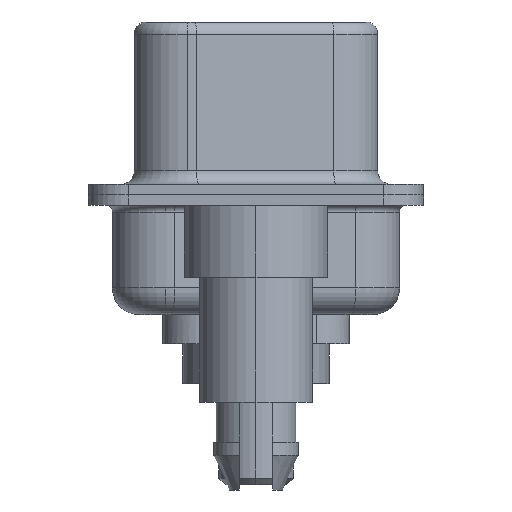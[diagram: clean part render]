
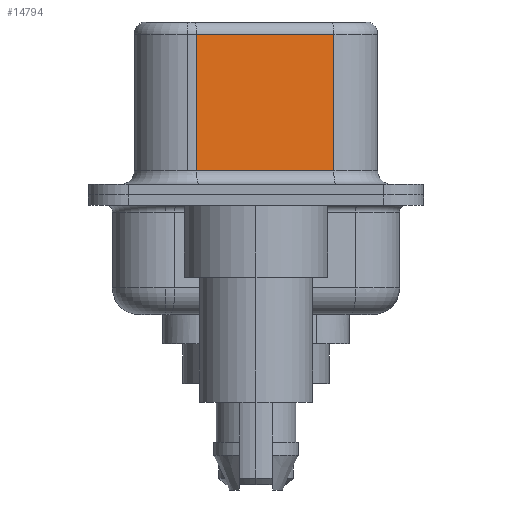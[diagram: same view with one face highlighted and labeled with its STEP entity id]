
A CAD part, left-side view. The second image highlights one B-rep face of the part: STEP entity #14794.
In plain terms, the highlighted planar face has unit normal (-0.985, -0.174, 0).
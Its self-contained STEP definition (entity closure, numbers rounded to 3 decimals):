
#834 = VECTOR ( 'NONE', #15636, 1000. ) ;
#1064 = VERTEX_POINT ( 'NONE', #4476 ) ;
#1557 = ORIENTED_EDGE ( 'NONE', *, *, #4398, .F. ) ;
#1974 = VECTOR ( 'NONE', #4565, 1000. ) ;
#2028 = VECTOR ( 'NONE', #15256, 1000. ) ;
#2409 = LINE ( 'NONE', #6386, #2028 ) ;
#4015 = CARTESIAN_POINT ( 'NONE',  ( 4.565, -2.927, 6.52 ) ) ;
#4229 = CARTESIAN_POINT ( 'NONE',  ( 3.655, 2.233, 6.02 ) ) ;
#4398 = EDGE_CURVE ( 'NONE', #12036, #6480, #5385, .T. ) ;
#4476 = CARTESIAN_POINT ( 'NONE',  ( 3.655, 2.233, 0.9 ) ) ;
#4565 = DIRECTION ( 'NONE',  ( 0., 0., -1. ) ) ;
#5288 = DIRECTION ( 'NONE',  ( 0.985, 0.174, 0. ) ) ;
#5385 = LINE ( 'NONE', #15519, #1974 ) ;
#5910 = CARTESIAN_POINT ( 'NONE',  ( 4.565, -2.927, 0.9 ) ) ;
#6386 = CARTESIAN_POINT ( 'NONE',  ( 4.565, -2.927, 0.9 ) ) ;
#6480 = VERTEX_POINT ( 'NONE', #5910 ) ;
#6602 = VERTEX_POINT ( 'NONE', #4229 ) ;
#7279 = LINE ( 'NONE', #13178, #834 ) ;
#7358 = CARTESIAN_POINT ( 'NONE',  ( 4.565, -2.927, 6.02 ) ) ;
#8392 = EDGE_LOOP ( 'NONE', ( #1557, #12049, #12335, #14996 ) ) ;
#9115 = LINE ( 'NONE', #14843, #12471 ) ;
#10158 = FACE_OUTER_BOUND ( 'NONE', #8392, .T. ) ;
#12036 = VERTEX_POINT ( 'NONE', #7358 ) ;
#12049 = ORIENTED_EDGE ( 'NONE', *, *, #13078, .T. ) ;
#12335 = ORIENTED_EDGE ( 'NONE', *, *, #12399, .T. ) ;
#12399 = EDGE_CURVE ( 'NONE', #6602, #1064, #7279, .T. ) ;
#12471 = VECTOR ( 'NONE', #16122, 1000. ) ;
#12948 = PLANE ( 'NONE',  #16230 ) ;
#13078 = EDGE_CURVE ( 'NONE', #12036, #6602, #9115, .T. ) ;
#13178 = CARTESIAN_POINT ( 'NONE',  ( 3.655, 2.233, 6.52 ) ) ;
#14169 = DIRECTION ( 'NONE',  ( -0.174, 0.985, 0. ) ) ;
#14794 = ADVANCED_FACE ( 'NONE', ( #10158 ), #12948, .F. ) ;
#14843 = CARTESIAN_POINT ( 'NONE',  ( 4.565, -2.927, 6.02 ) ) ;
#14996 = ORIENTED_EDGE ( 'NONE', *, *, #15460, .T. ) ;
#15256 = DIRECTION ( 'NONE',  ( 0.174, -0.985, 0. ) ) ;
#15460 = EDGE_CURVE ( 'NONE', #1064, #6480, #2409, .T. ) ;
#15519 = CARTESIAN_POINT ( 'NONE',  ( 4.565, -2.927, 6.52 ) ) ;
#15636 = DIRECTION ( 'NONE',  ( 0., 0., -1. ) ) ;
#16122 = DIRECTION ( 'NONE',  ( -0.174, 0.985, 0. ) ) ;
#16230 = AXIS2_PLACEMENT_3D ( 'NONE', #4015, #5288, #14169 ) ;
